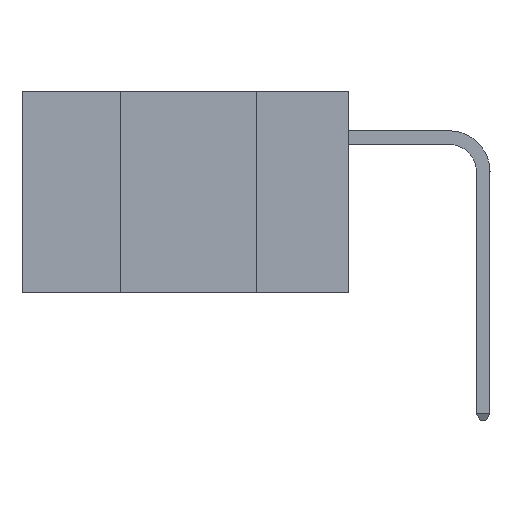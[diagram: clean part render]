
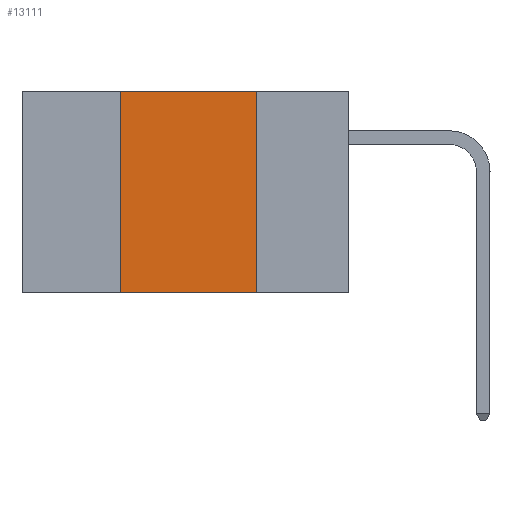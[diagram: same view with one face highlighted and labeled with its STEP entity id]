
A CAD part, left-side view. The second image highlights one B-rep face of the part: STEP entity #13111.
In plain terms, the highlighted planar face has unit normal (-1, 0, 0).
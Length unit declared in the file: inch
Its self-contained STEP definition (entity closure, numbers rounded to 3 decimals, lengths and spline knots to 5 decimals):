
#172 = VERTEX_POINT ( 'NONE', #7557 ) ;
#1210 = ORIENTED_EDGE ( 'NONE', *, *, #7546, .F. ) ;
#1915 = ORIENTED_EDGE ( 'NONE', *, *, #15626, .F. ) ;
#2605 = EDGE_CURVE ( 'NONE', #7977, #14243, #10029, .T. ) ;
#3591 = VECTOR ( 'NONE', #12171, 39.37008 ) ;
#4460 = VECTOR ( 'NONE', #19071, 39.37008 ) ;
#4606 = VECTOR ( 'NONE', #8343, 39.37008 ) ;
#5511 = FACE_OUTER_BOUND ( 'NONE', #17501, .T. ) ;
#6263 = VERTEX_POINT ( 'NONE', #16286 ) ;
#7095 = DIRECTION ( 'NONE',  ( 0., -1., 0. ) ) ;
#7546 = EDGE_CURVE ( 'NONE', #6263, #7977, #21614, .T. ) ;
#7557 = CARTESIAN_POINT ( 'NONE',  ( 0., 0.17, -0.37 ) ) ;
#7977 = VERTEX_POINT ( 'NONE', #11369 ) ;
#8111 = AXIS2_PLACEMENT_3D ( 'NONE', #20474, #11609, #27313 ) ;
#8343 = DIRECTION ( 'NONE',  ( 0., -1., 0. ) ) ;
#10029 = LINE ( 'NONE', #20558, #26516 ) ;
#11369 = CARTESIAN_POINT ( 'NONE',  ( 0., 0.42, 0. ) ) ;
#11609 = DIRECTION ( 'NONE',  ( 1., 0., 0. ) ) ;
#12171 = DIRECTION ( 'NONE',  ( 0., 0., 1. ) ) ;
#12473 = CARTESIAN_POINT ( 'NONE',  ( 0., 0.17, 0. ) ) ;
#13111 = ADVANCED_FACE ( 'NONE', ( #5511 ), #25049, .F. ) ;
#14243 = VERTEX_POINT ( 'NONE', #22108 ) ;
#14407 = CARTESIAN_POINT ( 'NONE',  ( 0., 0.42, 0. ) ) ;
#14522 = ORIENTED_EDGE ( 'NONE', *, *, #19167, .T. ) ;
#15626 = EDGE_CURVE ( 'NONE', #14243, #172, #16491, .T. ) ;
#16286 = CARTESIAN_POINT ( 'NONE',  ( 0., 0.42, -0.37 ) ) ;
#16491 = LINE ( 'NONE', #12473, #4460 ) ;
#16630 = LINE ( 'NONE', #26310, #4606 ) ;
#17501 = EDGE_LOOP ( 'NONE', ( #1915, #19080, #1210, #14522 ) ) ;
#19071 = DIRECTION ( 'NONE',  ( 0., 0., -1. ) ) ;
#19080 = ORIENTED_EDGE ( 'NONE', *, *, #2605, .F. ) ;
#19167 = EDGE_CURVE ( 'NONE', #6263, #172, #16630, .T. ) ;
#20474 = CARTESIAN_POINT ( 'NONE',  ( 0., 0.6, 0. ) ) ;
#20558 = CARTESIAN_POINT ( 'NONE',  ( 0., 0.6, 0. ) ) ;
#21614 = LINE ( 'NONE', #14407, #3591 ) ;
#22108 = CARTESIAN_POINT ( 'NONE',  ( 0., 0.17, 0. ) ) ;
#25049 = PLANE ( 'NONE',  #8111 ) ;
#26310 = CARTESIAN_POINT ( 'NONE',  ( 0., 0.6, -0.37 ) ) ;
#26516 = VECTOR ( 'NONE', #7095, 39.37008 ) ;
#27313 = DIRECTION ( 'NONE',  ( 0., 0., -1. ) ) ;
